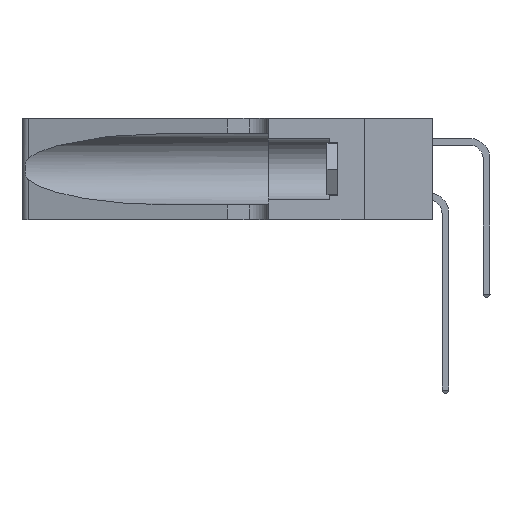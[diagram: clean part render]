
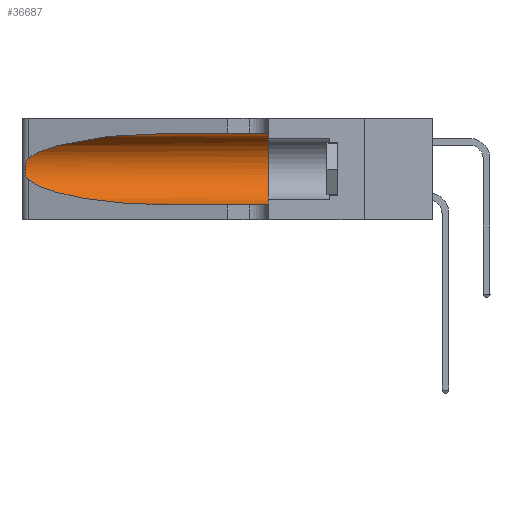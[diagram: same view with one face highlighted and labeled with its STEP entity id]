
A CAD part, left-side view. The second image highlights one B-rep face of the part: STEP entity #36687.
In plain terms, the highlighted cylindrical face has radius 3.308 mm (diameter 6.617 mm), a partial arc.
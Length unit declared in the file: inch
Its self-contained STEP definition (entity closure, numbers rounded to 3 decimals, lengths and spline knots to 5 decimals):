
#369 = DIRECTION ( 'NONE',  ( 0., -1., 0. ) ) ;
#1107 = ORIENTED_EDGE ( 'NONE', *, *, #25859, .T. ) ;
#1163 = ORIENTED_EDGE ( 'NONE', *, *, #40849, .T. ) ;
#1885 = DIRECTION ( 'NONE',  ( 0., -1., 0. ) ) ;
#2683 = AXIS2_PLACEMENT_3D ( 'NONE', #17813, #369, #21159 ) ;
#2965 = CARTESIAN_POINT ( 'NONE',  ( 0.25487, 1.22718, 0.22369 ) ) ;
#3122 = CARTESIAN_POINT ( 'NONE',  ( 0.25487, 1.22718, 0.14631 ) ) ;
#4351 = EDGE_CURVE ( 'NONE', #21425, #36813, #16049, .T. ) ;
#4872 = CARTESIAN_POINT ( 'NONE',  ( 0.2373, 1.15595, 0.28018 ) ) ;
#5741 = CARTESIAN_POINT ( 'NONE',  ( 0.25487, 1.22718, 0.14631 ) ) ;
#5847 = ORIENTED_EDGE ( 'NONE', *, *, #4351, .T. ) ;
#6472 = CARTESIAN_POINT ( 'NONE',  ( 0.25639, 1.23184, 0.21858 ) ) ;
#9115 = VECTOR ( 'NONE', #11982, 39.37008 ) ;
#9983 = CARTESIAN_POINT ( 'NONE',  ( 0.25854, 1.2359, 0.20912 ) ) ;
#11333 = EDGE_CURVE ( 'NONE', #21425, #15892, #17166, .T. ) ;
#11486 = VERTEX_POINT ( 'NONE', #5741 ) ;
#11982 = DIRECTION ( 'NONE',  ( 0., -1., 0. ) ) ;
#13454 = CARTESIAN_POINT ( 'NONE',  ( 0.26075, 1.23896, 0.19203 ) ) ;
#14070 = DIRECTION ( 'NONE',  ( 0., 1., 0. ) ) ;
#15341 = CARTESIAN_POINT ( 'NONE',  ( 0.25487, 1.22718, 0.22369 ) ) ;
#15892 = VERTEX_POINT ( 'NONE', #31424 ) ;
#16011 = CYLINDRICAL_SURFACE ( 'NONE', #2683, 0.13025 ) ;
#16049 =( BOUNDED_CURVE ( )  B_SPLINE_CURVE ( 3, ( #35296, #28630, #4872, #15341 ),
 .UNSPECIFIED., .F., .F. ) 
 B_SPLINE_CURVE_WITH_KNOTS ( ( 4, 4 ),
 ( 1.5708, 2.84003 ),
 .UNSPECIFIED. ) 
 CURVE ( )  GEOMETRIC_REPRESENTATION_ITEM ( )  RATIONAL_B_SPLINE_CURVE ( ( 1., 0.87, 0.87, 1. ) ) 
 REPRESENTATION_ITEM ( '' )  );
#16868 = CARTESIAN_POINT ( 'NONE',  ( 0.26017, 1.23833, 0.17102 ) ) ;
#17166 = LINE ( 'NONE', #42019, #9115 ) ;
#17813 = CARTESIAN_POINT ( 'NONE',  ( 0.1305, 1.61858, 0.185 ) ) ;
#17897 = VERTEX_POINT ( 'NONE', #32140 ) ;
#18365 = VECTOR ( 'NONE', #1885, 39.37008 ) ;
#18375 = EDGE_LOOP ( 'NONE', ( #5847, #1107, #1163, #39423, #28699, #40543 ) ) ;
#18566 = CARTESIAN_POINT ( 'NONE',  ( 0.1305, 0.72297, 0.05475 ) ) ;
#20219 = CARTESIAN_POINT ( 'NONE',  ( 0.25789, 1.23486, 0.15765 ) ) ;
#21023 = EDGE_CURVE ( 'NONE', #15892, #17897, #39631, .T. ) ;
#21159 = DIRECTION ( 'NONE',  ( 0., 0., -1. ) ) ;
#21425 = VERTEX_POINT ( 'NONE', #39300 ) ;
#21750 = CARTESIAN_POINT ( 'NONE',  ( 0.25487, 1.22718, 0.14631 ) ) ;
#22407 = CARTESIAN_POINT ( 'NONE',  ( 0.1305, 1.61858, 0.05475 ) ) ;
#23554 = VERTEX_POINT ( 'NONE', #37905 ) ;
#23579 = CARTESIAN_POINT ( 'NONE',  ( 0.25555, 1.22993, 0.14849 ) ) ;
#25134 = B_SPLINE_CURVE_WITH_KNOTS ( 'NONE', 3,
 ( #2965, #26814, #6472, #30131, #9983, #33498, #13454, #36832, #16868, #40215, #20219, #43580, #23579, #3122 ),
 .UNSPECIFIED., .F., .F.,
 ( 4, 2, 2, 2, 2, 2, 4 ),
 ( 0., 0.00027, 0.00053, 0.00107, 0.0016, 0.00187, 0.00214 ),
 .UNSPECIFIED. ) ;
#25859 = EDGE_CURVE ( 'NONE', #36813, #11486, #25134, .T. ) ;
#26223 = LINE ( 'NONE', #22407, #18365 ) ;
#26814 = CARTESIAN_POINT ( 'NONE',  ( 0.25555, 1.22994, 0.2215 ) ) ;
#28630 = CARTESIAN_POINT ( 'NONE',  ( 0.18966, 0.96281, 0.31525 ) ) ;
#28699 = ORIENTED_EDGE ( 'NONE', *, *, #21023, .F. ) ;
#29700 =( BOUNDED_CURVE ( )  B_SPLINE_CURVE ( 3, ( #21750, #35144, #38540, #18566 ),
 .UNSPECIFIED., .F., .F. ) 
 B_SPLINE_CURVE_WITH_KNOTS ( ( 4, 4 ),
 ( 3.44316, 4.71239 ),
 .UNSPECIFIED. ) 
 CURVE ( )  GEOMETRIC_REPRESENTATION_ITEM ( )  RATIONAL_B_SPLINE_CURVE ( ( 1., 0.87, 0.87, 1. ) ) 
 REPRESENTATION_ITEM ( '' )  );
#30131 = CARTESIAN_POINT ( 'NONE',  ( 0.25787, 1.23484, 0.2124 ) ) ;
#31424 = CARTESIAN_POINT ( 'NONE',  ( 0.1305, 0.35, 0.31525 ) ) ;
#32140 = CARTESIAN_POINT ( 'NONE',  ( 0.1305, 0.35, 0.05475 ) ) ;
#32397 = CARTESIAN_POINT ( 'NONE',  ( 0.25487, 1.22718, 0.22369 ) ) ;
#33195 = EDGE_CURVE ( 'NONE', #23554, #17897, #26223, .T. ) ;
#33498 = CARTESIAN_POINT ( 'NONE',  ( 0.26018, 1.23835, 0.19895 ) ) ;
#34058 = CARTESIAN_POINT ( 'NONE',  ( 0.1305, 0.35, 0.185 ) ) ;
#35144 = CARTESIAN_POINT ( 'NONE',  ( 0.2373, 1.15595, 0.08982 ) ) ;
#35296 = CARTESIAN_POINT ( 'NONE',  ( 0.1305, 0.72297, 0.31525 ) ) ;
#36687 = ADVANCED_FACE ( 'NONE', ( #42684 ), #16011, .F. ) ;
#36813 = VERTEX_POINT ( 'NONE', #32397 ) ;
#36832 = CARTESIAN_POINT ( 'NONE',  ( 0.26075, 1.23896, 0.178 ) ) ;
#37432 = DIRECTION ( 'NONE',  ( 0., 0., 1. ) ) ;
#37905 = CARTESIAN_POINT ( 'NONE',  ( 0.1305, 0.72297, 0.05475 ) ) ;
#38540 = CARTESIAN_POINT ( 'NONE',  ( 0.18966, 0.96281, 0.05475 ) ) ;
#39300 = CARTESIAN_POINT ( 'NONE',  ( 0.1305, 0.72297, 0.31525 ) ) ;
#39423 = ORIENTED_EDGE ( 'NONE', *, *, #33195, .T. ) ;
#39631 = CIRCLE ( 'NONE', #40802, 0.13025 ) ;
#40215 = CARTESIAN_POINT ( 'NONE',  ( 0.25856, 1.23593, 0.16098 ) ) ;
#40543 = ORIENTED_EDGE ( 'NONE', *, *, #11333, .F. ) ;
#40802 = AXIS2_PLACEMENT_3D ( 'NONE', #34058, #14070, #37432 ) ;
#40849 = EDGE_CURVE ( 'NONE', #11486, #23554, #29700, .T. ) ;
#42019 = CARTESIAN_POINT ( 'NONE',  ( 0.1305, 1.61858, 0.31525 ) ) ;
#42684 = FACE_OUTER_BOUND ( 'NONE', #18375, .T. ) ;
#43580 = CARTESIAN_POINT ( 'NONE',  ( 0.25639, 1.23186, 0.15144 ) ) ;
